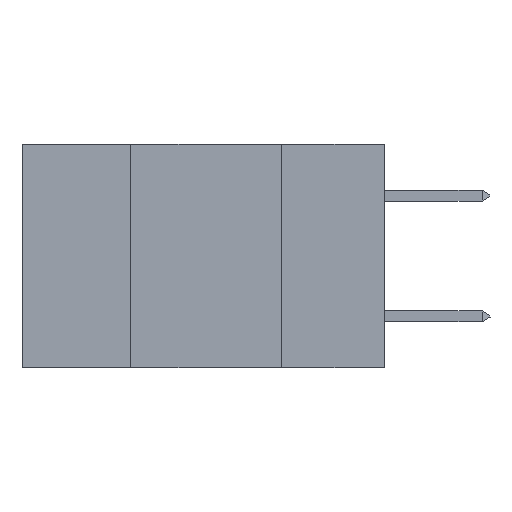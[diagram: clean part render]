
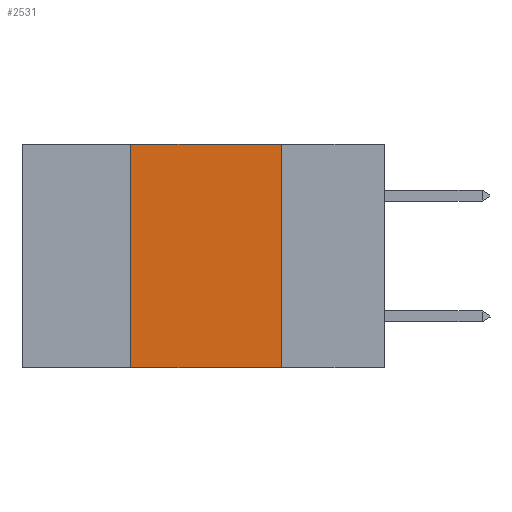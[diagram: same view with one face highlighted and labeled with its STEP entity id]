
A CAD part, left-side view. The second image highlights one B-rep face of the part: STEP entity #2531.
In plain terms, the highlighted planar face has unit normal (-1, 0, 0).
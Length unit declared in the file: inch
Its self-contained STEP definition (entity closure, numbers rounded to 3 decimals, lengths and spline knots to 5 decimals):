
#283 = EDGE_CURVE ( 'NONE', #3781, #16923, #5746, .T. ) ;
#325 = ORIENTED_EDGE ( 'NONE', *, *, #283, .T. ) ;
#2531 = ADVANCED_FACE ( 'NONE', ( #15729 ), #18992, .F. ) ;
#3781 = VERTEX_POINT ( 'NONE', #30359 ) ;
#4158 = VECTOR ( 'NONE', #22960, 39.37008 ) ;
#4336 = CARTESIAN_POINT ( 'NONE',  ( 0., 0.6, -0.37 ) ) ;
#5746 = LINE ( 'NONE', #4336, #34345 ) ;
#5901 = ORIENTED_EDGE ( 'NONE', *, *, #30614, .F. ) ;
#7880 = DIRECTION ( 'NONE',  ( 0., -1., 0. ) ) ;
#7899 = CARTESIAN_POINT ( 'NONE',  ( 0., 0.6, 0. ) ) ;
#8379 = CARTESIAN_POINT ( 'NONE',  ( 0., 0.42, 0. ) ) ;
#10605 = LINE ( 'NONE', #8379, #25730 ) ;
#10805 = DIRECTION ( 'NONE',  ( 0., 0., 1. ) ) ;
#10967 = CARTESIAN_POINT ( 'NONE',  ( 0., 0.42, 0. ) ) ;
#11499 = VERTEX_POINT ( 'NONE', #11997 ) ;
#11997 = CARTESIAN_POINT ( 'NONE',  ( 0., 0.17, 0. ) ) ;
#13038 = EDGE_LOOP ( 'NONE', ( #23799, #5901, #31799, #325 ) ) ;
#13783 = LINE ( 'NONE', #30241, #25050 ) ;
#15729 = FACE_OUTER_BOUND ( 'NONE', #13038, .T. ) ;
#16923 = VERTEX_POINT ( 'NONE', #24868 ) ;
#17474 = CARTESIAN_POINT ( 'NONE',  ( 0., 0.17, 0. ) ) ;
#18992 = PLANE ( 'NONE',  #21842 ) ;
#21842 = AXIS2_PLACEMENT_3D ( 'NONE', #7899, #35272, #27278 ) ;
#22960 = DIRECTION ( 'NONE',  ( 0., 0., -1. ) ) ;
#23799 = ORIENTED_EDGE ( 'NONE', *, *, #26300, .F. ) ;
#24868 = CARTESIAN_POINT ( 'NONE',  ( 0., 0.17, -0.37 ) ) ;
#25050 = VECTOR ( 'NONE', #7880, 39.37008 ) ;
#25730 = VECTOR ( 'NONE', #10805, 39.37008 ) ;
#26300 = EDGE_CURVE ( 'NONE', #11499, #16923, #32792, .T. ) ;
#27057 = DIRECTION ( 'NONE',  ( 0., -1., 0. ) ) ;
#27278 = DIRECTION ( 'NONE',  ( 0., 0., -1. ) ) ;
#27510 = EDGE_CURVE ( 'NONE', #3781, #28099, #10605, .T. ) ;
#28099 = VERTEX_POINT ( 'NONE', #10967 ) ;
#30241 = CARTESIAN_POINT ( 'NONE',  ( 0., 0.6, 0. ) ) ;
#30359 = CARTESIAN_POINT ( 'NONE',  ( 0., 0.42, -0.37 ) ) ;
#30614 = EDGE_CURVE ( 'NONE', #28099, #11499, #13783, .T. ) ;
#31799 = ORIENTED_EDGE ( 'NONE', *, *, #27510, .F. ) ;
#32792 = LINE ( 'NONE', #17474, #4158 ) ;
#34345 = VECTOR ( 'NONE', #27057, 39.37008 ) ;
#35272 = DIRECTION ( 'NONE',  ( 1., 0., 0. ) ) ;
